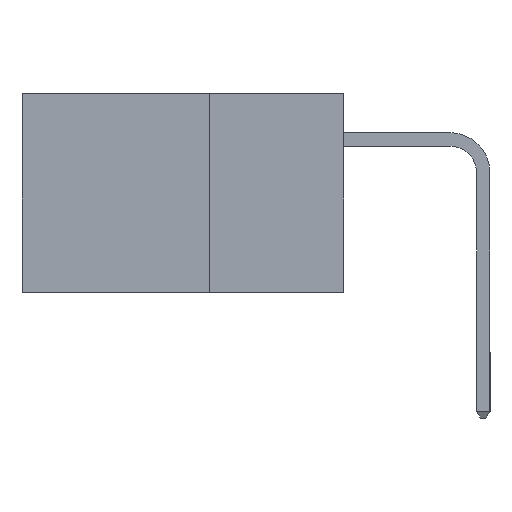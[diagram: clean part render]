
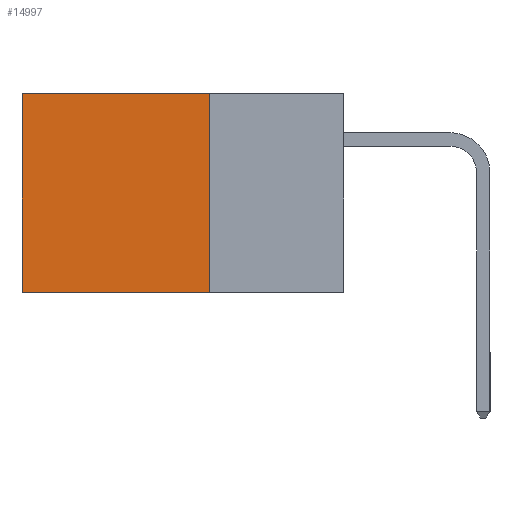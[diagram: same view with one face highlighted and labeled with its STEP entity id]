
A CAD part, left-side view. The second image highlights one B-rep face of the part: STEP entity #14997.
In plain terms, the highlighted planar face has unit normal (-1, 0, 0).
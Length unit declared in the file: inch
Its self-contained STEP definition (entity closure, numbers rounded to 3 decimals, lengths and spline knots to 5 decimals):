
#710 = DIRECTION ( 'NONE',  ( 0., 1., 0. ) ) ;
#1033 = VECTOR ( 'NONE', #20305, 39.37008 ) ;
#1154 = ORIENTED_EDGE ( 'NONE', *, *, #15924, .T. ) ;
#2558 = CARTESIAN_POINT ( 'NONE',  ( 0.298, 0.25, 0. ) ) ;
#3124 = CARTESIAN_POINT ( 'NONE',  ( 0.298, 0.6, 0. ) ) ;
#3620 = EDGE_CURVE ( 'NONE', #14226, #4614, #6806, .T. ) ;
#4614 = VERTEX_POINT ( 'NONE', #9288 ) ;
#4627 = CARTESIAN_POINT ( 'NONE',  ( 0.298, 0.6, -0.37 ) ) ;
#4902 = DIRECTION ( 'NONE',  ( 0., 0., -1. ) ) ;
#4995 = CARTESIAN_POINT ( 'NONE',  ( 0.298, 0.25, 0. ) ) ;
#6472 = VECTOR ( 'NONE', #9535, 39.37008 ) ;
#6806 = LINE ( 'NONE', #4995, #9221 ) ;
#7735 = CARTESIAN_POINT ( 'NONE',  ( 0.298, 0.25, -0.37 ) ) ;
#9221 = VECTOR ( 'NONE', #16518, 39.37008 ) ;
#9288 = CARTESIAN_POINT ( 'NONE',  ( 0.298, 0.25, -0.37 ) ) ;
#9535 = DIRECTION ( 'NONE',  ( 0., 0., -1. ) ) ;
#9931 = CARTESIAN_POINT ( 'NONE',  ( 0.298, 0.6, 0. ) ) ;
#10257 = EDGE_CURVE ( 'NONE', #14226, #11059, #18125, .T. ) ;
#10699 = VERTEX_POINT ( 'NONE', #4627 ) ;
#11059 = VERTEX_POINT ( 'NONE', #9931 ) ;
#13416 = PLANE ( 'NONE',  #20809 ) ;
#13691 = EDGE_LOOP ( 'NONE', ( #1154, #15461, #27201, #14053 ) ) ;
#14053 = ORIENTED_EDGE ( 'NONE', *, *, #10257, .T. ) ;
#14226 = VERTEX_POINT ( 'NONE', #24350 ) ;
#14997 = ADVANCED_FACE ( 'NONE', ( #28733 ), #13416, .F. ) ;
#15461 = ORIENTED_EDGE ( 'NONE', *, *, #23003, .F. ) ;
#15924 = EDGE_CURVE ( 'NONE', #11059, #10699, #24870, .T. ) ;
#16518 = DIRECTION ( 'NONE',  ( 0., 0., -1. ) ) ;
#17211 = LINE ( 'NONE', #7735, #20336 ) ;
#18125 = LINE ( 'NONE', #26680, #1033 ) ;
#20305 = DIRECTION ( 'NONE',  ( 0., 1., 0. ) ) ;
#20336 = VECTOR ( 'NONE', #710, 39.37008 ) ;
#20809 = AXIS2_PLACEMENT_3D ( 'NONE', #2558, #24697, #4902 ) ;
#23003 = EDGE_CURVE ( 'NONE', #4614, #10699, #17211, .T. ) ;
#24350 = CARTESIAN_POINT ( 'NONE',  ( 0.298, 0.25, 0. ) ) ;
#24697 = DIRECTION ( 'NONE',  ( 1., 0., 0. ) ) ;
#24870 = LINE ( 'NONE', #3124, #6472 ) ;
#26680 = CARTESIAN_POINT ( 'NONE',  ( 0.298, 0.25, 0. ) ) ;
#27201 = ORIENTED_EDGE ( 'NONE', *, *, #3620, .F. ) ;
#28733 = FACE_OUTER_BOUND ( 'NONE', #13691, .T. ) ;
